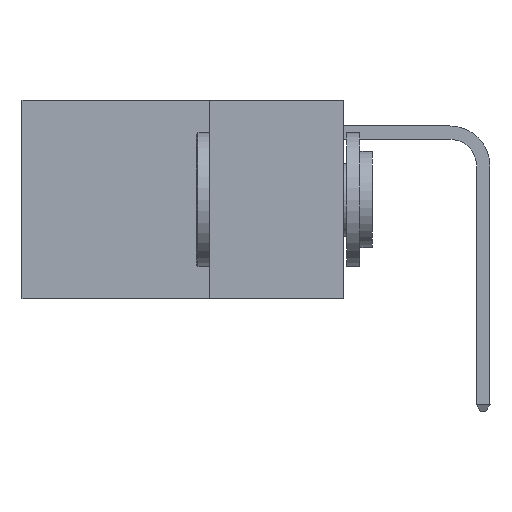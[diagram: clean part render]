
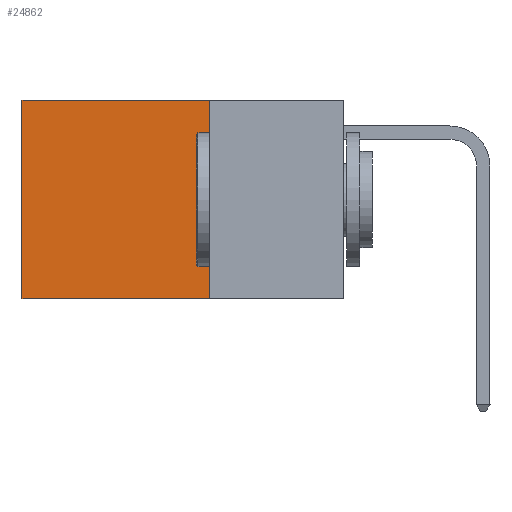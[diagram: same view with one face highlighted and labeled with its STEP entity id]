
A CAD part, left-side view. The second image highlights one B-rep face of the part: STEP entity #24862.
In plain terms, the highlighted planar face has unit normal (-1, 0, 0).
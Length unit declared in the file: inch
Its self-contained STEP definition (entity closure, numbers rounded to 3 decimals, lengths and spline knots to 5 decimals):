
#1941 = CARTESIAN_POINT ( 'NONE',  ( 0.2625, 0.6, 0. ) ) ;
#2502 = DIRECTION ( 'NONE',  ( 0., 0., -1. ) ) ;
#2861 = CARTESIAN_POINT ( 'NONE',  ( 0.2625, 0.6, 0. ) ) ;
#3613 = EDGE_CURVE ( 'NONE', #15409, #15758, #14131, .T. ) ;
#4214 = VECTOR ( 'NONE', #11874, 39.37008 ) ;
#5113 = CARTESIAN_POINT ( 'NONE',  ( 0.2625, 0.6, -0.37 ) ) ;
#6036 = VECTOR ( 'NONE', #2502, 39.37008 ) ;
#7484 = FACE_OUTER_BOUND ( 'NONE', #27994, .T. ) ;
#7734 = CARTESIAN_POINT ( 'NONE',  ( 0.2625, 0.25, 0. ) ) ;
#7886 = EDGE_CURVE ( 'NONE', #14419, #13091, #22528, .T. ) ;
#8045 = CARTESIAN_POINT ( 'NONE',  ( 0.2625, 0.25, -0.37 ) ) ;
#9107 = ORIENTED_EDGE ( 'NONE', *, *, #24945, .T. ) ;
#9276 = VECTOR ( 'NONE', #22850, 39.37008 ) ;
#9891 = VECTOR ( 'NONE', #22189, 39.37008 ) ;
#10455 = LINE ( 'NONE', #8045, #9276 ) ;
#11874 = DIRECTION ( 'NONE',  ( 0., 0., -1. ) ) ;
#12009 = DIRECTION ( 'NONE',  ( 1., 0., 0. ) ) ;
#13091 = VERTEX_POINT ( 'NONE', #5113 ) ;
#13981 = CARTESIAN_POINT ( 'NONE',  ( 0.2625, 0.25, 0. ) ) ;
#14131 = LINE ( 'NONE', #13981, #4214 ) ;
#14419 = VERTEX_POINT ( 'NONE', #2861 ) ;
#15409 = VERTEX_POINT ( 'NONE', #7734 ) ;
#15758 = VERTEX_POINT ( 'NONE', #23416 ) ;
#17108 = AXIS2_PLACEMENT_3D ( 'NONE', #19375, #12009, #21169 ) ;
#18314 = ORIENTED_EDGE ( 'NONE', *, *, #25347, .F. ) ;
#19375 = CARTESIAN_POINT ( 'NONE',  ( 0.2625, 0.25, 0. ) ) ;
#21169 = DIRECTION ( 'NONE',  ( 0., 0., -1. ) ) ;
#21467 = PLANE ( 'NONE',  #17108 ) ;
#22189 = DIRECTION ( 'NONE',  ( 0., 1., 0. ) ) ;
#22528 = LINE ( 'NONE', #1941, #6036 ) ;
#22850 = DIRECTION ( 'NONE',  ( 0., 1., 0. ) ) ;
#23297 = ORIENTED_EDGE ( 'NONE', *, *, #7886, .T. ) ;
#23416 = CARTESIAN_POINT ( 'NONE',  ( 0.2625, 0.25, -0.37 ) ) ;
#24862 = ADVANCED_FACE ( 'NONE', ( #7484 ), #21467, .F. ) ;
#24945 = EDGE_CURVE ( 'NONE', #15409, #14419, #29082, .T. ) ;
#25347 = EDGE_CURVE ( 'NONE', #15758, #13091, #10455, .T. ) ;
#27127 = CARTESIAN_POINT ( 'NONE',  ( 0.2625, 0.25, 0. ) ) ;
#27994 = EDGE_LOOP ( 'NONE', ( #23297, #18314, #29547, #9107 ) ) ;
#29082 = LINE ( 'NONE', #27127, #9891 ) ;
#29547 = ORIENTED_EDGE ( 'NONE', *, *, #3613, .F. ) ;
